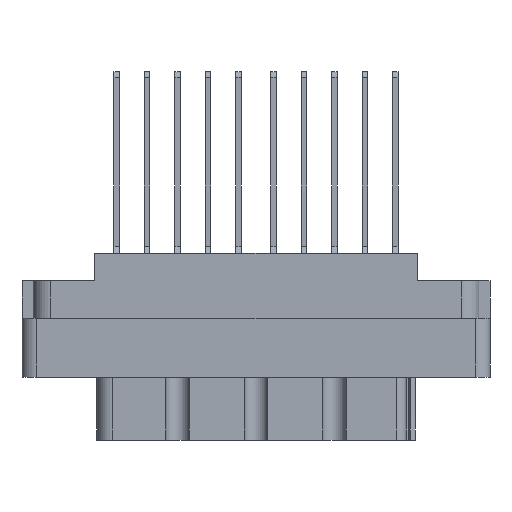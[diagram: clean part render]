
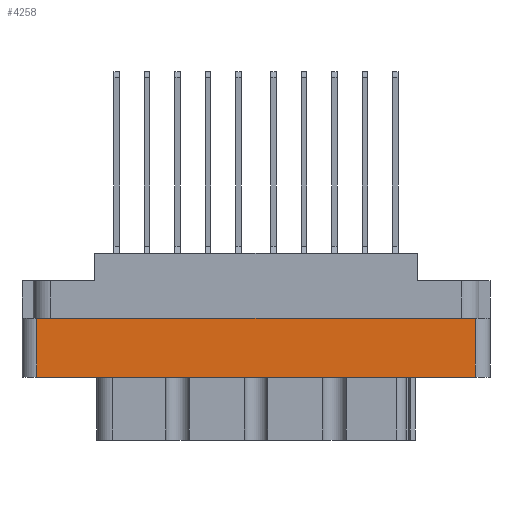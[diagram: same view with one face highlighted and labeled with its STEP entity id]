
A CAD part, front view. The second image highlights one B-rep face of the part: STEP entity #4258.
In plain terms, the highlighted planar face has unit normal (0, -1, 0).
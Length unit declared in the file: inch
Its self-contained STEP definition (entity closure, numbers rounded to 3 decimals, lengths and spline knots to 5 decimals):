
#1592 = ORIENTED_EDGE ( 'NONE', *, *, #18317, .T. ) ;
#4258 = ADVANCED_FACE ( 'NONE', ( #32053 ), #8509, .T. ) ;
#6477 = CARTESIAN_POINT ( 'NONE',  ( -0.938, -0.438, -0.277 ) ) ;
#8201 = VERTEX_POINT ( 'NONE', #29531 ) ;
#8509 = PLANE ( 'NONE',  #11266 ) ;
#9102 = EDGE_CURVE ( 'NONE', #18790, #9118, #16084, .T. ) ;
#9118 = VERTEX_POINT ( 'NONE', #21180 ) ;
#9417 = DIRECTION ( 'NONE',  ( -1., 0., 0. ) ) ;
#10790 = VECTOR ( 'NONE', #25892, 39.37008 ) ;
#11233 = LINE ( 'NONE', #28550, #12228 ) ;
#11266 = AXIS2_PLACEMENT_3D ( 'NONE', #26762, #27030, #20568 ) ;
#11603 = ORIENTED_EDGE ( 'NONE', *, *, #13759, .F. ) ;
#12228 = VECTOR ( 'NONE', #19495, 39.37008 ) ;
#13759 = EDGE_CURVE ( 'NONE', #18790, #8201, #21188, .T. ) ;
#14754 = DIRECTION ( 'NONE',  ( 0., 0., 1. ) ) ;
#16084 = LINE ( 'NONE', #23934, #23654 ) ;
#18317 = EDGE_CURVE ( 'NONE', #27340, #8201, #31456, .T. ) ;
#18775 = EDGE_CURVE ( 'NONE', #27340, #9118, #11233, .T. ) ;
#18790 = VERTEX_POINT ( 'NONE', #34598 ) ;
#19495 = DIRECTION ( 'NONE',  ( 1., 0., 0. ) ) ;
#19508 = ORIENTED_EDGE ( 'NONE', *, *, #18775, .F. ) ;
#20568 = DIRECTION ( 'NONE',  ( 0., 0., -1. ) ) ;
#21180 = CARTESIAN_POINT ( 'NONE',  ( 0.938, -0.438, -0.277 ) ) ;
#21188 = LINE ( 'NONE', #36068, #33404 ) ;
#22854 = CARTESIAN_POINT ( 'NONE',  ( -0.938, -0.438, -0.798 ) ) ;
#23654 = VECTOR ( 'NONE', #14754, 39.37008 ) ;
#23934 = CARTESIAN_POINT ( 'NONE',  ( 0.938, -0.438, -0.798 ) ) ;
#25111 = EDGE_LOOP ( 'NONE', ( #19508, #1592, #11603, #37240 ) ) ;
#25892 = DIRECTION ( 'NONE',  ( 0., 0., -1. ) ) ;
#26762 = CARTESIAN_POINT ( 'NONE',  ( -1., -0.438, -0.798 ) ) ;
#27030 = DIRECTION ( 'NONE',  ( 0., -1., 0. ) ) ;
#27340 = VERTEX_POINT ( 'NONE', #6477 ) ;
#28550 = CARTESIAN_POINT ( 'NONE',  ( 0., -0.438, -0.277 ) ) ;
#29531 = CARTESIAN_POINT ( 'NONE',  ( -0.938, -0.438, -0.529 ) ) ;
#31456 = LINE ( 'NONE', #22854, #10790 ) ;
#32053 = FACE_OUTER_BOUND ( 'NONE', #25111, .T. ) ;
#33404 = VECTOR ( 'NONE', #9417, 39.37008 ) ;
#34598 = CARTESIAN_POINT ( 'NONE',  ( 0.938, -0.438, -0.529 ) ) ;
#36068 = CARTESIAN_POINT ( 'NONE',  ( 0., -0.438, -0.529 ) ) ;
#37240 = ORIENTED_EDGE ( 'NONE', *, *, #9102, .T. ) ;
